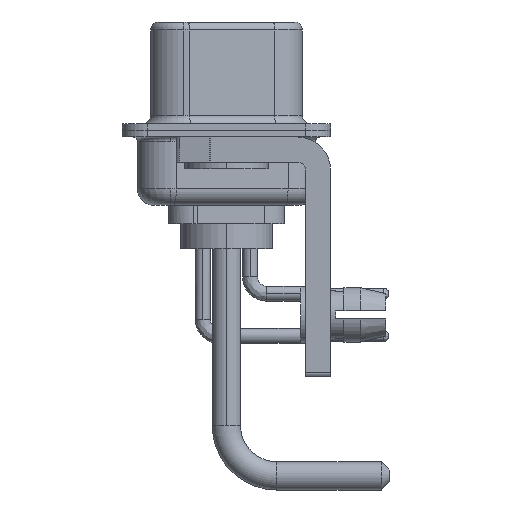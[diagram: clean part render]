
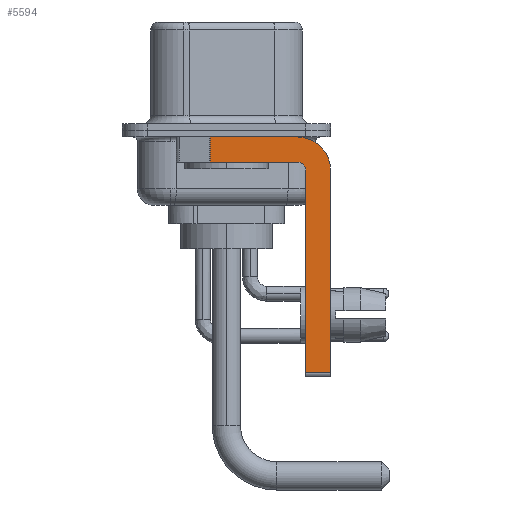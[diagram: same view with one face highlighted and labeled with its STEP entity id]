
A CAD part, left-side view. The second image highlights one B-rep face of the part: STEP entity #5594.
In plain terms, the highlighted planar face has unit normal (-1, 0, 0).
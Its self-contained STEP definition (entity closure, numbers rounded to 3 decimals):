
#425 = EDGE_CURVE ( 'NONE', #23497, #9037, #6201, .T. ) ;
#1508 = VECTOR ( 'NONE', #17893, 1000. ) ;
#1511 = VECTOR ( 'NONE', #22265, 1000. ) ;
#1944 = CARTESIAN_POINT ( 'NONE',  ( -2.9, -4.75, -14.8 ) ) ;
#2184 = CARTESIAN_POINT ( 'NONE',  ( -2.9, -6.25, -14.55 ) ) ;
#2408 = CIRCLE ( 'NONE', #10914, 0.5 ) ;
#2463 = DIRECTION ( 'NONE',  ( 1., 0., 0. ) ) ;
#2900 = CARTESIAN_POINT ( 'NONE',  ( -2.9, -4.25, -1.9 ) ) ;
#3946 = VERTEX_POINT ( 'NONE', #2184 ) ;
#5594 = ADVANCED_FACE ( 'NONE', ( #23907 ), #8260, .F. ) ;
#6163 = VERTEX_POINT ( 'NONE', #18264 ) ;
#6201 = CIRCLE ( 'NONE', #22672, 2. ) ;
#6215 = DIRECTION ( 'NONE',  ( 0., 0., -1. ) ) ;
#6372 = DIRECTION ( 'NONE',  ( 0., -1., 0. ) ) ;
#8260 = PLANE ( 'NONE',  #21008 ) ;
#8969 = ORIENTED_EDGE ( 'NONE', *, *, #22619, .F. ) ;
#9023 = DIRECTION ( 'NONE',  ( 0., 0., 1. ) ) ;
#9037 = VERTEX_POINT ( 'NONE', #25365 ) ;
#9097 = DIRECTION ( 'NONE',  ( 0., 1., 0. ) ) ;
#9199 = ORIENTED_EDGE ( 'NONE', *, *, #17808, .F. ) ;
#9235 = ORIENTED_EDGE ( 'NONE', *, *, #23075, .F. ) ;
#9260 = LINE ( 'NONE', #13530, #1511 ) ;
#9695 = DIRECTION ( 'NONE',  ( 0., 0., -1. ) ) ;
#9939 = EDGE_CURVE ( 'NONE', #26588, #6163, #15728, .T. ) ;
#9984 = VECTOR ( 'NONE', #9023, 1000. ) ;
#10772 = CARTESIAN_POINT ( 'NONE',  ( -2.9, -4.25, -2.4 ) ) ;
#10914 = AXIS2_PLACEMENT_3D ( 'NONE', #17133, #21859, #21274 ) ;
#10926 = ORIENTED_EDGE ( 'NONE', *, *, #425, .F. ) ;
#10950 = LINE ( 'NONE', #1944, #9984 ) ;
#11528 = EDGE_CURVE ( 'NONE', #13947, #3946, #14745, .T. ) ;
#11907 = VECTOR ( 'NONE', #6372, 1000. ) ;
#12179 = ORIENTED_EDGE ( 'NONE', *, *, #21593, .F. ) ;
#12990 = CARTESIAN_POINT ( 'NONE',  ( -2.9, -4.75, -2.4 ) ) ;
#13530 = CARTESIAN_POINT ( 'NONE',  ( -2.9, 0.978, -1.9 ) ) ;
#13947 = VERTEX_POINT ( 'NONE', #26966 ) ;
#14151 = DIRECTION ( 'NONE',  ( 0., -1., 0. ) ) ;
#14745 = LINE ( 'NONE', #16809, #16475 ) ;
#15728 = LINE ( 'NONE', #20300, #19683 ) ;
#15881 = CARTESIAN_POINT ( 'NONE',  ( -2.9, -4.25, -2.4 ) ) ;
#16475 = VECTOR ( 'NONE', #14151, 1000. ) ;
#16726 = ORIENTED_EDGE ( 'NONE', *, *, #11528, .T. ) ;
#16809 = CARTESIAN_POINT ( 'NONE',  ( -2.9, -4.25, -14.55 ) ) ;
#17133 = CARTESIAN_POINT ( 'NONE',  ( -2.9, -4.25, -2.4 ) ) ;
#17504 = CARTESIAN_POINT ( 'NONE',  ( -2.9, 0.978, -0.4 ) ) ;
#17808 = EDGE_CURVE ( 'NONE', #13947, #24759, #10950, .T. ) ;
#17893 = DIRECTION ( 'NONE',  ( 0., 0., -1. ) ) ;
#18249 = ORIENTED_EDGE ( 'NONE', *, *, #9939, .F. ) ;
#18264 = CARTESIAN_POINT ( 'NONE',  ( -2.9, 0.978, -1.9 ) ) ;
#19683 = VECTOR ( 'NONE', #9097, 1000. ) ;
#19967 = CARTESIAN_POINT ( 'NONE',  ( -2.9, -6.25, -2.4 ) ) ;
#20300 = CARTESIAN_POINT ( 'NONE',  ( -2.9, -4.25, -1.9 ) ) ;
#21008 = AXIS2_PLACEMENT_3D ( 'NONE', #10772, #21689, #6215 ) ;
#21274 = DIRECTION ( 'NONE',  ( 0., 0., 1. ) ) ;
#21593 = EDGE_CURVE ( 'NONE', #24759, #26588, #2408, .T. ) ;
#21689 = DIRECTION ( 'NONE',  ( 1., 0., 0. ) ) ;
#21859 = DIRECTION ( 'NONE',  ( -1., 0., 0. ) ) ;
#22004 = LINE ( 'NONE', #28797, #11907 ) ;
#22265 = DIRECTION ( 'NONE',  ( 0., 0., -1. ) ) ;
#22619 = EDGE_CURVE ( 'NONE', #9037, #3946, #28686, .T. ) ;
#22672 = AXIS2_PLACEMENT_3D ( 'NONE', #15881, #2463, #9695 ) ;
#23075 = EDGE_CURVE ( 'NONE', #29086, #23497, #22004, .T. ) ;
#23497 = VERTEX_POINT ( 'NONE', #24598 ) ;
#23907 = FACE_OUTER_BOUND ( 'NONE', #25235, .T. ) ;
#24598 = CARTESIAN_POINT ( 'NONE',  ( -2.9, -4.25, -0.4 ) ) ;
#24759 = VERTEX_POINT ( 'NONE', #12990 ) ;
#25235 = EDGE_LOOP ( 'NONE', ( #9235, #29024, #18249, #12179, #9199, #16726, #8969, #10926 ) ) ;
#25365 = CARTESIAN_POINT ( 'NONE',  ( -2.9, -6.25, -2.4 ) ) ;
#26588 = VERTEX_POINT ( 'NONE', #2900 ) ;
#26966 = CARTESIAN_POINT ( 'NONE',  ( -2.9, -4.75, -14.55 ) ) ;
#27459 = EDGE_CURVE ( 'NONE', #29086, #6163, #9260, .T. ) ;
#28686 = LINE ( 'NONE', #19967, #1508 ) ;
#28797 = CARTESIAN_POINT ( 'NONE',  ( -2.9, 3., -0.4 ) ) ;
#29024 = ORIENTED_EDGE ( 'NONE', *, *, #27459, .T. ) ;
#29086 = VERTEX_POINT ( 'NONE', #17504 ) ;
